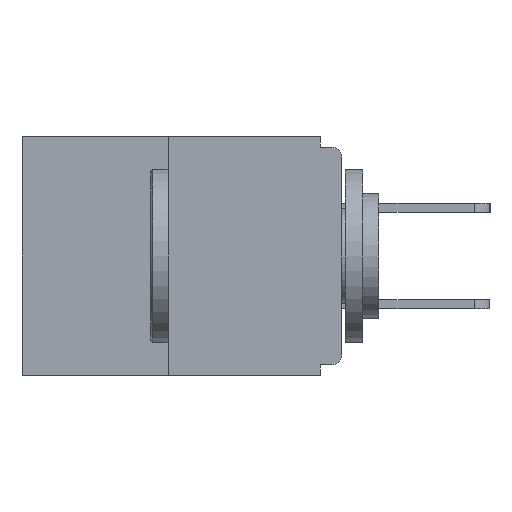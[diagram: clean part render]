
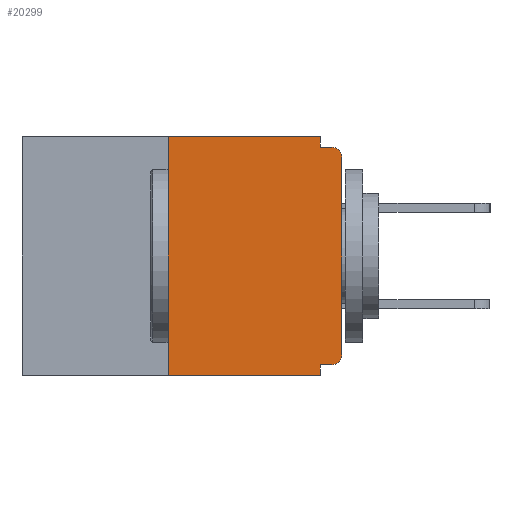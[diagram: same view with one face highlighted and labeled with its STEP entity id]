
A CAD part, left-side view. The second image highlights one B-rep face of the part: STEP entity #20299.
In plain terms, the highlighted planar face has unit normal (-1, 0, 0).
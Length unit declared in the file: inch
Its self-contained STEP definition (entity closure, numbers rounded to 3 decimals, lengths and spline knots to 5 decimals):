
#143 = CARTESIAN_POINT ( 'NONE',  ( 0., 0.015, -0.015 ) ) ;
#427 = CARTESIAN_POINT ( 'NONE',  ( 0., 0.031, -0.343 ) ) ;
#956 = EDGE_CURVE ( 'NONE', #22187, #1546, #3836, .T. ) ;
#1128 = LINE ( 'NONE', #4443, #22798 ) ;
#1188 = CARTESIAN_POINT ( 'NONE',  ( 0., 0.015, -0.313 ) ) ;
#1377 = EDGE_LOOP ( 'NONE', ( #21643, #3468, #13995, #17445, #14202, #17386, #21700, #13269, #25981, #21683 ) ) ;
#1454 = DIRECTION ( 'NONE',  ( -1., 0., 0. ) ) ;
#1546 = VERTEX_POINT ( 'NONE', #20021 ) ;
#1708 = VERTEX_POINT ( 'NONE', #22810 ) ;
#2288 = EDGE_CURVE ( 'NONE', #9787, #8287, #1128, .T. ) ;
#2335 = VECTOR ( 'NONE', #20114, 39.37008 ) ;
#2588 = DIRECTION ( 'NONE',  ( 0., -1., 0. ) ) ;
#2710 = VECTOR ( 'NONE', #6368, 39.37008 ) ;
#2780 = CARTESIAN_POINT ( 'NONE',  ( 0., 0.015, -0.03 ) ) ;
#3291 = CARTESIAN_POINT ( 'NONE',  ( 0., 0.25, 0. ) ) ;
#3468 = ORIENTED_EDGE ( 'NONE', *, *, #22422, .F. ) ;
#3730 = EDGE_CURVE ( 'NONE', #12214, #20247, #25989, .T. ) ;
#3836 = LINE ( 'NONE', #20136, #7423 ) ;
#4102 = CARTESIAN_POINT ( 'NONE',  ( 0., 0.031, -0.015 ) ) ;
#4261 = CIRCLE ( 'NONE', #22023, 0.015 ) ;
#4443 = CARTESIAN_POINT ( 'NONE',  ( 0., 0.46, -0.343 ) ) ;
#4905 = DIRECTION ( 'NONE',  ( 0., 0., -1. ) ) ;
#5023 = CARTESIAN_POINT ( 'NONE',  ( 0., 0.46, 0. ) ) ;
#6368 = DIRECTION ( 'NONE',  ( 0., -1., 0. ) ) ;
#6549 = CARTESIAN_POINT ( 'NONE',  ( 0., 0., -0.313 ) ) ;
#6677 = VERTEX_POINT ( 'NONE', #4102 ) ;
#6766 = LINE ( 'NONE', #8224, #21127 ) ;
#7141 = DIRECTION ( 'NONE',  ( 0., 0., -1. ) ) ;
#7423 = VECTOR ( 'NONE', #18052, 39.37008 ) ;
#7637 = VERTEX_POINT ( 'NONE', #24924 ) ;
#8224 = CARTESIAN_POINT ( 'NONE',  ( 0., 0.031, 0. ) ) ;
#8287 = VERTEX_POINT ( 'NONE', #12433 ) ;
#8981 = VECTOR ( 'NONE', #11847, 39.37008 ) ;
#9787 = VERTEX_POINT ( 'NONE', #15423 ) ;
#10138 = CARTESIAN_POINT ( 'NONE',  ( 0., 0.015, -0.328 ) ) ;
#10260 = VECTOR ( 'NONE', #13809, 39.37008 ) ;
#11609 = PLANE ( 'NONE',  #23895 ) ;
#11829 = DIRECTION ( 'NONE',  ( 0., 0., -1. ) ) ;
#11847 = DIRECTION ( 'NONE',  ( 0., -1., 0. ) ) ;
#12214 = VERTEX_POINT ( 'NONE', #10138 ) ;
#12433 = CARTESIAN_POINT ( 'NONE',  ( 0., 0.031, -0.343 ) ) ;
#12582 = LINE ( 'NONE', #427, #20736 ) ;
#12790 = VERTEX_POINT ( 'NONE', #143 ) ;
#13269 = ORIENTED_EDGE ( 'NONE', *, *, #25985, .T. ) ;
#13682 = DIRECTION ( 'NONE',  ( 1., 0., 0. ) ) ;
#13809 = DIRECTION ( 'NONE',  ( 0., 1., 0. ) ) ;
#13995 = ORIENTED_EDGE ( 'NONE', *, *, #2288, .T. ) ;
#14048 = EDGE_CURVE ( 'NONE', #12214, #22187, #14977, .T. ) ;
#14202 = ORIENTED_EDGE ( 'NONE', *, *, #3730, .F. ) ;
#14977 = CIRCLE ( 'NONE', #17841, 0.015 ) ;
#15313 = CARTESIAN_POINT ( 'NONE',  ( 0., 0., -0.328 ) ) ;
#15423 = CARTESIAN_POINT ( 'NONE',  ( 0., 0.25, -0.343 ) ) ;
#16082 = EDGE_CURVE ( 'NONE', #7637, #1708, #21697, .T. ) ;
#16105 = EDGE_CURVE ( 'NONE', #6677, #12790, #22356, .T. ) ;
#17386 = ORIENTED_EDGE ( 'NONE', *, *, #14048, .T. ) ;
#17445 = ORIENTED_EDGE ( 'NONE', *, *, #20183, .F. ) ;
#17841 = AXIS2_PLACEMENT_3D ( 'NONE', #1188, #1454, #11829 ) ;
#18052 = DIRECTION ( 'NONE',  ( 0., 0., 1. ) ) ;
#19406 = EDGE_CURVE ( 'NONE', #1708, #6677, #6766, .T. ) ;
#19466 = CARTESIAN_POINT ( 'NONE',  ( 0., 0.031, -0.328 ) ) ;
#19747 = FACE_OUTER_BOUND ( 'NONE', #1377, .T. ) ;
#20021 = CARTESIAN_POINT ( 'NONE',  ( 0., 0., -0.03 ) ) ;
#20114 = DIRECTION ( 'NONE',  ( 0., 0., 1. ) ) ;
#20136 = CARTESIAN_POINT ( 'NONE',  ( 0., 0., 0. ) ) ;
#20183 = EDGE_CURVE ( 'NONE', #20247, #8287, #12582, .T. ) ;
#20247 = VERTEX_POINT ( 'NONE', #19466 ) ;
#20299 = ADVANCED_FACE ( 'NONE', ( #19747 ), #11609, .F. ) ;
#20656 = LINE ( 'NONE', #3291, #2335 ) ;
#20736 = VECTOR ( 'NONE', #21474, 39.37008 ) ;
#21127 = VECTOR ( 'NONE', #23510, 39.37008 ) ;
#21474 = DIRECTION ( 'NONE',  ( 0., 0., -1. ) ) ;
#21643 = ORIENTED_EDGE ( 'NONE', *, *, #16082, .F. ) ;
#21683 = ORIENTED_EDGE ( 'NONE', *, *, #19406, .F. ) ;
#21697 = LINE ( 'NONE', #24411, #8981 ) ;
#21700 = ORIENTED_EDGE ( 'NONE', *, *, #956, .T. ) ;
#22023 = AXIS2_PLACEMENT_3D ( 'NONE', #2780, #23420, #4905 ) ;
#22187 = VERTEX_POINT ( 'NONE', #6549 ) ;
#22356 = LINE ( 'NONE', #25053, #2710 ) ;
#22422 = EDGE_CURVE ( 'NONE', #9787, #7637, #20656, .T. ) ;
#22798 = VECTOR ( 'NONE', #2588, 39.37008 ) ;
#22810 = CARTESIAN_POINT ( 'NONE',  ( 0., 0.031, 0. ) ) ;
#23420 = DIRECTION ( 'NONE',  ( -1., 0., 0. ) ) ;
#23510 = DIRECTION ( 'NONE',  ( 0., 0., -1. ) ) ;
#23895 = AXIS2_PLACEMENT_3D ( 'NONE', #5023, #13682, #7141 ) ;
#24411 = CARTESIAN_POINT ( 'NONE',  ( 0., 0.46, 0. ) ) ;
#24924 = CARTESIAN_POINT ( 'NONE',  ( 0., 0.25, 0. ) ) ;
#25053 = CARTESIAN_POINT ( 'NONE',  ( 0., 0., -0.015 ) ) ;
#25981 = ORIENTED_EDGE ( 'NONE', *, *, #16105, .F. ) ;
#25985 = EDGE_CURVE ( 'NONE', #1546, #12790, #4261, .T. ) ;
#25989 = LINE ( 'NONE', #15313, #10260 ) ;
